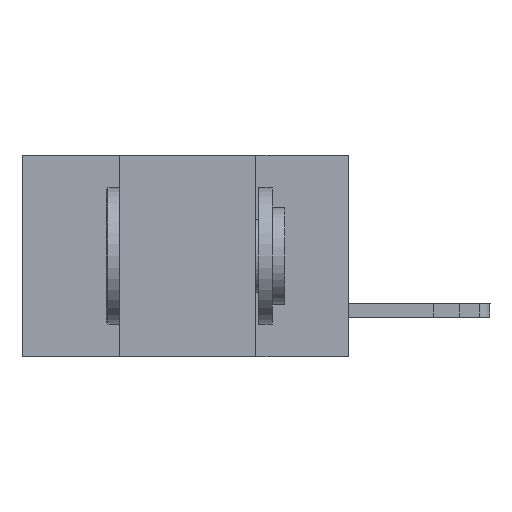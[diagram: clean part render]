
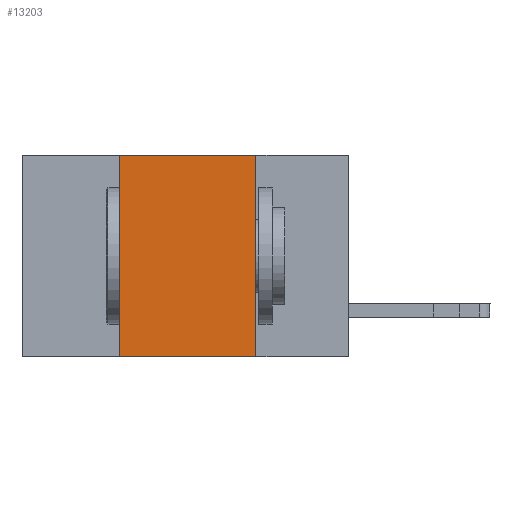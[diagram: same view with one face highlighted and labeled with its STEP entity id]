
A CAD part, left-side view. The second image highlights one B-rep face of the part: STEP entity #13203.
In plain terms, the highlighted planar face has unit normal (-1, 0, 0).
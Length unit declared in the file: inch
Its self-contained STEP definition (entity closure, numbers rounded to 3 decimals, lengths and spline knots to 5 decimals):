
#2086 = DIRECTION ( 'NONE',  ( 0., 0., -1. ) ) ;
#2133 = CARTESIAN_POINT ( 'NONE',  ( 0., 0.17, 0. ) ) ;
#3256 = EDGE_LOOP ( 'NONE', ( #15164, #21297, #14250, #18639 ) ) ;
#4084 = CARTESIAN_POINT ( 'NONE',  ( 0., 0.42, -0.37 ) ) ;
#5009 = EDGE_CURVE ( 'NONE', #16625, #9535, #12275, .T. ) ;
#5304 = CARTESIAN_POINT ( 'NONE',  ( 0., 0.6, 0. ) ) ;
#7038 = CARTESIAN_POINT ( 'NONE',  ( 0., 0.42, -0.37 ) ) ;
#7096 = PLANE ( 'NONE',  #15268 ) ;
#7281 = DIRECTION ( 'NONE',  ( 0., -1., 0. ) ) ;
#9535 = VERTEX_POINT ( 'NONE', #21067 ) ;
#10135 = VERTEX_POINT ( 'NONE', #11822 ) ;
#10326 = CARTESIAN_POINT ( 'NONE',  ( 0., 0.6, 0. ) ) ;
#10757 = VECTOR ( 'NONE', #7281, 39.37008 ) ;
#10965 = VECTOR ( 'NONE', #15809, 39.37008 ) ;
#11431 = DIRECTION ( 'NONE',  ( 0., -1., 0. ) ) ;
#11822 = CARTESIAN_POINT ( 'NONE',  ( 0., 0.42, 0. ) ) ;
#12149 = DIRECTION ( 'NONE',  ( 1., 0., 0. ) ) ;
#12275 = LINE ( 'NONE', #19034, #12366 ) ;
#12366 = VECTOR ( 'NONE', #2086, 39.37008 ) ;
#12892 = CARTESIAN_POINT ( 'NONE',  ( 0., 0.6, -0.37 ) ) ;
#13203 = ADVANCED_FACE ( 'NONE', ( #20591 ), #7096, .F. ) ;
#13237 = EDGE_CURVE ( 'NONE', #14046, #10135, #21345, .T. ) ;
#13868 = EDGE_CURVE ( 'NONE', #14046, #9535, #16310, .T. ) ;
#14046 = VERTEX_POINT ( 'NONE', #7038 ) ;
#14250 = ORIENTED_EDGE ( 'NONE', *, *, #13237, .F. ) ;
#15164 = ORIENTED_EDGE ( 'NONE', *, *, #5009, .F. ) ;
#15268 = AXIS2_PLACEMENT_3D ( 'NONE', #5304, #12149, #18917 ) ;
#15809 = DIRECTION ( 'NONE',  ( 0., 0., 1. ) ) ;
#16310 = LINE ( 'NONE', #12892, #18804 ) ;
#16625 = VERTEX_POINT ( 'NONE', #2133 ) ;
#17333 = LINE ( 'NONE', #10326, #10757 ) ;
#18639 = ORIENTED_EDGE ( 'NONE', *, *, #13868, .T. ) ;
#18804 = VECTOR ( 'NONE', #11431, 39.37008 ) ;
#18917 = DIRECTION ( 'NONE',  ( 0., 0., -1. ) ) ;
#19034 = CARTESIAN_POINT ( 'NONE',  ( 0., 0.17, -0.37 ) ) ;
#19313 = EDGE_CURVE ( 'NONE', #10135, #16625, #17333, .T. ) ;
#20591 = FACE_OUTER_BOUND ( 'NONE', #3256, .T. ) ;
#21067 = CARTESIAN_POINT ( 'NONE',  ( 0., 0.17, -0.37 ) ) ;
#21297 = ORIENTED_EDGE ( 'NONE', *, *, #19313, .F. ) ;
#21345 = LINE ( 'NONE', #4084, #10965 ) ;
